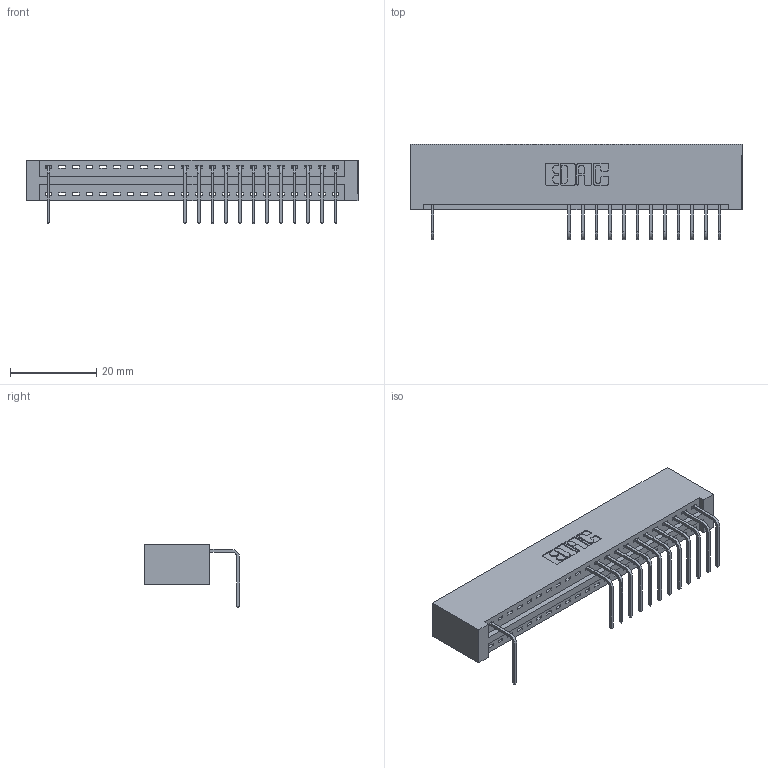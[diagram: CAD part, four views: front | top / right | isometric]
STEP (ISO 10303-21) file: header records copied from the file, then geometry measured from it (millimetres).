
FILE_DESCRIPTION (( 'STEP AP203' ), '1' );
FILE_NAME ('346-022-558-101.STEP', '2018-08-21T01:01:53', ( '' ), ( '' ), 'SwSTEP 2.0', 'SolidWorks 2016', '' );
FILE_SCHEMA (( 'CONFIG_CONTROL_DESIGN' ));
Length unit declared in the file: inch
Products named in the file (3): 346 Part_No Mounting Lugs; 345-292-001_558 Tail - 2; 346-022-558-101
Assembly tree (14 placements, depth 2):
  346-022-558-101
    346 Part_No Mounting Lugs
    345-292-001_558 Tail - 2  x13
Bounding box: 77.09 x 22.16 x 14.73 mm (x, y, z)
Volume: 7731.1 mm3; surface area: 9226.8 mm2
Topology: 14 solids, 14 shells, 1002 faces, 3049 edges, 2014 vertices
Faces by surface type: plane 708, cylinder 294
Entity records: 15865 total; most frequent: CARTESIAN_POINT 2773, ORIENTED_EDGE 2738, DIRECTION 2455, EDGE_CURVE 1369, LINE 1157, VECTOR 1157, VERTEX_POINT 910, AXIS2_PLACEMENT_3D 649
